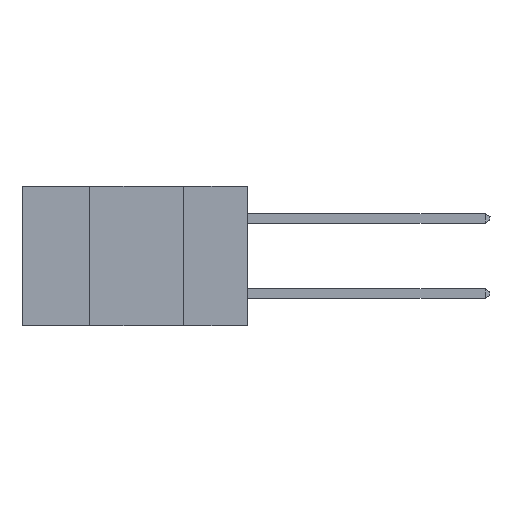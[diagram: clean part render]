
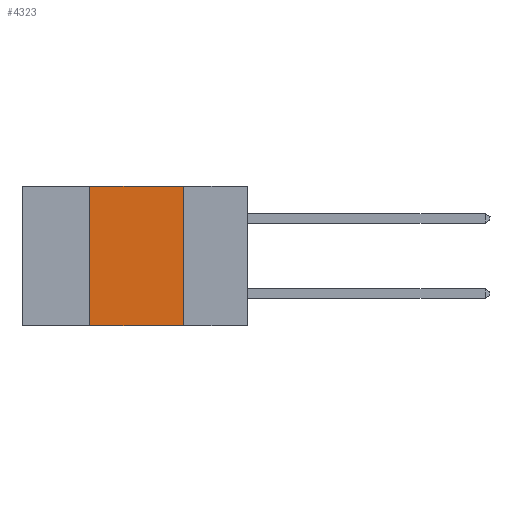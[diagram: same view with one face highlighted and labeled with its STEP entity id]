
A CAD part, left-side view. The second image highlights one B-rep face of the part: STEP entity #4323.
In plain terms, the highlighted planar face has unit normal (-1, 0, 0).
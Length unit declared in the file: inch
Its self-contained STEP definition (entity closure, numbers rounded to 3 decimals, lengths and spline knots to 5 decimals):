
#140 = CARTESIAN_POINT ( 'NONE',  ( 0., 0.42, 0. ) ) ;
#611 = ORIENTED_EDGE ( 'NONE', *, *, #6885, .T. ) ;
#1013 = LINE ( 'NONE', #9965, #11987 ) ;
#1800 = VERTEX_POINT ( 'NONE', #3007 ) ;
#2198 = DIRECTION ( 'NONE',  ( 0., 0., -1. ) ) ;
#2528 = EDGE_LOOP ( 'NONE', ( #9345, #3172, #11733, #611 ) ) ;
#3007 = CARTESIAN_POINT ( 'NONE',  ( 0., 0.17, -0.37 ) ) ;
#3172 = ORIENTED_EDGE ( 'NONE', *, *, #10486, .F. ) ;
#4139 = VECTOR ( 'NONE', #8995, 39.37008 ) ;
#4323 = ADVANCED_FACE ( 'NONE', ( #13851 ), #8976, .F. ) ;
#4475 = DIRECTION ( 'NONE',  ( 1., 0., 0. ) ) ;
#5494 = EDGE_CURVE ( 'NONE', #7935, #1800, #8289, .T. ) ;
#5869 = AXIS2_PLACEMENT_3D ( 'NONE', #7892, #4475, #2198 ) ;
#6678 = DIRECTION ( 'NONE',  ( 0., 0., -1. ) ) ;
#6885 = EDGE_CURVE ( 'NONE', #11287, #1800, #1013, .T. ) ;
#7247 = VECTOR ( 'NONE', #6678, 39.37008 ) ;
#7821 = DIRECTION ( 'NONE',  ( 0., -1., 0. ) ) ;
#7892 = CARTESIAN_POINT ( 'NONE',  ( 0., 0.6, 0. ) ) ;
#7935 = VERTEX_POINT ( 'NONE', #14211 ) ;
#7958 = CARTESIAN_POINT ( 'NONE',  ( 0., 0.42, 0. ) ) ;
#8289 = LINE ( 'NONE', #13547, #7247 ) ;
#8976 = PLANE ( 'NONE',  #5869 ) ;
#8995 = DIRECTION ( 'NONE',  ( 0., 0., 1. ) ) ;
#9095 = CARTESIAN_POINT ( 'NONE',  ( 0., 0.42, -0.37 ) ) ;
#9114 = VERTEX_POINT ( 'NONE', #140 ) ;
#9345 = ORIENTED_EDGE ( 'NONE', *, *, #5494, .F. ) ;
#9965 = CARTESIAN_POINT ( 'NONE',  ( 0., 0.6, -0.37 ) ) ;
#10486 = EDGE_CURVE ( 'NONE', #9114, #7935, #11155, .T. ) ;
#11155 = LINE ( 'NONE', #14637, #14339 ) ;
#11287 = VERTEX_POINT ( 'NONE', #9095 ) ;
#11733 = ORIENTED_EDGE ( 'NONE', *, *, #12954, .F. ) ;
#11967 = LINE ( 'NONE', #7958, #4139 ) ;
#11987 = VECTOR ( 'NONE', #7821, 39.37008 ) ;
#12245 = DIRECTION ( 'NONE',  ( 0., -1., 0. ) ) ;
#12954 = EDGE_CURVE ( 'NONE', #11287, #9114, #11967, .T. ) ;
#13547 = CARTESIAN_POINT ( 'NONE',  ( 0., 0.17, 0. ) ) ;
#13851 = FACE_OUTER_BOUND ( 'NONE', #2528, .T. ) ;
#14211 = CARTESIAN_POINT ( 'NONE',  ( 0., 0.17, 0. ) ) ;
#14339 = VECTOR ( 'NONE', #12245, 39.37008 ) ;
#14637 = CARTESIAN_POINT ( 'NONE',  ( 0., 0.6, 0. ) ) ;
